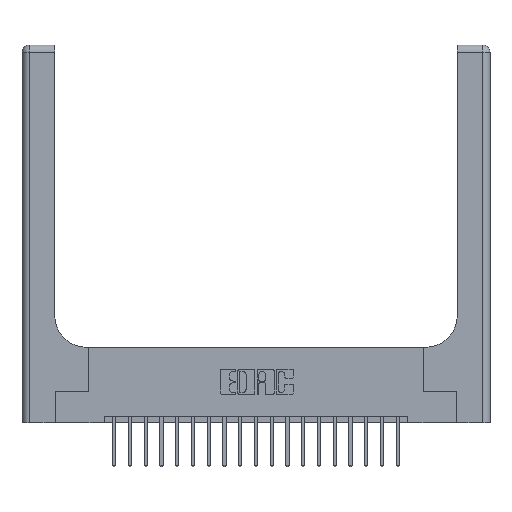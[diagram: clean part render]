
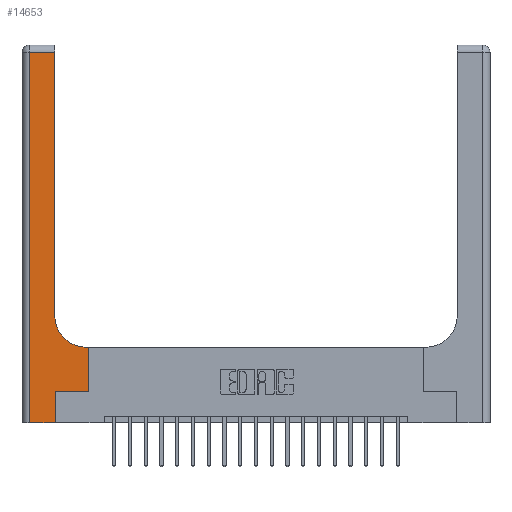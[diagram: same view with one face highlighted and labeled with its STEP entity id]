
A CAD part, top view. The second image highlights one B-rep face of the part: STEP entity #14653.
In plain terms, the highlighted planar face has unit normal (0, 0, 1).
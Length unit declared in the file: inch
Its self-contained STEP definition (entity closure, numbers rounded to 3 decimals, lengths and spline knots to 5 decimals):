
#74 = ORIENTED_EDGE ( 'NONE', *, *, #16744, .T. ) ;
#78 = AXIS2_PLACEMENT_3D ( 'NONE', #3815, #18214, #10391 ) ;
#103 = ORIENTED_EDGE ( 'NONE', *, *, #17492, .T. ) ;
#240 = VERTEX_POINT ( 'NONE', #12959 ) ;
#319 = CARTESIAN_POINT ( 'NONE',  ( 0., 3., 0.37 ) ) ;
#432 = LINE ( 'NONE', #9106, #1951 ) ;
#448 = ORIENTED_EDGE ( 'NONE', *, *, #4448, .T. ) ;
#1082 = ORIENTED_EDGE ( 'NONE', *, *, #11368, .T. ) ;
#1351 = CARTESIAN_POINT ( 'NONE',  ( 0.528, 0.25, 0.37 ) ) ;
#1389 = CARTESIAN_POINT ( 'NONE',  ( 0.06, 3., 0.37 ) ) ;
#1571 = CARTESIAN_POINT ( 'NONE',  ( 0.51, 0.6, 0.37 ) ) ;
#1824 = EDGE_CURVE ( 'NONE', #19904, #15926, #9438, .T. ) ;
#1832 = ORIENTED_EDGE ( 'NONE', *, *, #1824, .T. ) ;
#1951 = VECTOR ( 'NONE', #10669, 39.37008 ) ;
#2538 = CARTESIAN_POINT ( 'NONE',  ( 0.26, 2.94, 0.37 ) ) ;
#3023 = VERTEX_POINT ( 'NONE', #7259 ) ;
#3669 = EDGE_CURVE ( 'NONE', #5647, #3811, #8363, .T. ) ;
#3811 = VERTEX_POINT ( 'NONE', #5288 ) ;
#3815 = CARTESIAN_POINT ( 'NONE',  ( 0.51, 0.85, 0.37 ) ) ;
#4448 = EDGE_CURVE ( 'NONE', #3023, #19904, #19360, .T. ) ;
#4745 = VERTEX_POINT ( 'NONE', #18680 ) ;
#4746 = DIRECTION ( 'NONE',  ( -1., 0., 0. ) ) ;
#4914 = DIRECTION ( 'NONE',  ( 0., 0., -1. ) ) ;
#5176 = CARTESIAN_POINT ( 'NONE',  ( 0.265, 0.25, 0.37 ) ) ;
#5288 = CARTESIAN_POINT ( 'NONE',  ( 0.06, 2.94, 0.37 ) ) ;
#5647 = VERTEX_POINT ( 'NONE', #2538 ) ;
#5693 = ORIENTED_EDGE ( 'NONE', *, *, #3669, .T. ) ;
#6535 = DIRECTION ( 'NONE',  ( -1., 0., 0. ) ) ;
#6679 = CARTESIAN_POINT ( 'NONE',  ( 0.528, 0.25, 0.37 ) ) ;
#6680 = LINE ( 'NONE', #14009, #18183 ) ;
#7118 = VECTOR ( 'NONE', #4746, 39.37008 ) ;
#7122 = VECTOR ( 'NONE', #7865, 39.37008 ) ;
#7259 = CARTESIAN_POINT ( 'NONE',  ( 0.265, 0.25, 0.37 ) ) ;
#7482 = VERTEX_POINT ( 'NONE', #10153 ) ;
#7650 = EDGE_CURVE ( 'NONE', #11487, #240, #10318, .T. ) ;
#7865 = DIRECTION ( 'NONE',  ( 0., -1., 0. ) ) ;
#8240 = FACE_OUTER_BOUND ( 'NONE', #15623, .T. ) ;
#8363 = LINE ( 'NONE', #9780, #7118 ) ;
#8425 = VECTOR ( 'NONE', #17927, 39.37008 ) ;
#9106 = CARTESIAN_POINT ( 'NONE',  ( 0.265, 0., 0.37 ) ) ;
#9153 = CARTESIAN_POINT ( 'NONE',  ( 0.26, 3., 0.37 ) ) ;
#9438 = LINE ( 'NONE', #6679, #12708 ) ;
#9780 = CARTESIAN_POINT ( 'NONE',  ( 0., 2.94, 0.37 ) ) ;
#10153 = CARTESIAN_POINT ( 'NONE',  ( 0.06, 0., 0.37 ) ) ;
#10318 = CIRCLE ( 'NONE', #78, 0.25 ) ;
#10391 = DIRECTION ( 'NONE',  ( 1., 0., 0. ) ) ;
#10669 = DIRECTION ( 'NONE',  ( 0., 1., 0. ) ) ;
#10756 = EDGE_CURVE ( 'NONE', #240, #5647, #19450, .T. ) ;
#11368 = EDGE_CURVE ( 'NONE', #4745, #3023, #432, .T. ) ;
#11487 = VERTEX_POINT ( 'NONE', #1571 ) ;
#11767 = CARTESIAN_POINT ( 'NONE',  ( 0.26, 0.6, 0.37 ) ) ;
#12708 = VECTOR ( 'NONE', #17800, 39.37008 ) ;
#12905 = AXIS2_PLACEMENT_3D ( 'NONE', #319, #4914, #6535 ) ;
#12959 = CARTESIAN_POINT ( 'NONE',  ( 0.26, 0.85, 0.37 ) ) ;
#14009 = CARTESIAN_POINT ( 'NONE',  ( 0., 0., 0.37 ) ) ;
#14226 = LINE ( 'NONE', #11767, #8425 ) ;
#14653 = ADVANCED_FACE ( 'NONE', ( #8240 ), #17858, .F. ) ;
#14669 = CARTESIAN_POINT ( 'NONE',  ( 0.528, 0.6, 0.37 ) ) ;
#15095 = VECTOR ( 'NONE', #19467, 39.37008 ) ;
#15248 = ORIENTED_EDGE ( 'NONE', *, *, #7650, .T. ) ;
#15623 = EDGE_LOOP ( 'NONE', ( #17321, #5693, #16428, #103, #1082, #448, #1832, #74, #15248 ) ) ;
#15887 = LINE ( 'NONE', #1389, #7122 ) ;
#15926 = VERTEX_POINT ( 'NONE', #14669 ) ;
#16428 = ORIENTED_EDGE ( 'NONE', *, *, #18263, .T. ) ;
#16744 = EDGE_CURVE ( 'NONE', #15926, #11487, #14226, .T. ) ;
#17071 = DIRECTION ( 'NONE',  ( 1., 0., 0. ) ) ;
#17321 = ORIENTED_EDGE ( 'NONE', *, *, #10756, .T. ) ;
#17492 = EDGE_CURVE ( 'NONE', #7482, #4745, #6680, .T. ) ;
#17800 = DIRECTION ( 'NONE',  ( 0., 1., 0. ) ) ;
#17858 = PLANE ( 'NONE',  #12905 ) ;
#17927 = DIRECTION ( 'NONE',  ( -1., 0., 0. ) ) ;
#18183 = VECTOR ( 'NONE', #17071, 39.37008 ) ;
#18214 = DIRECTION ( 'NONE',  ( 0., 0., -1. ) ) ;
#18263 = EDGE_CURVE ( 'NONE', #3811, #7482, #15887, .T. ) ;
#18680 = CARTESIAN_POINT ( 'NONE',  ( 0.265, 0., 0.37 ) ) ;
#18823 = DIRECTION ( 'NONE',  ( 0., 1., 0. ) ) ;
#19360 = LINE ( 'NONE', #5176, #15095 ) ;
#19450 = LINE ( 'NONE', #9153, #20686 ) ;
#19467 = DIRECTION ( 'NONE',  ( 1., 0., 0. ) ) ;
#19904 = VERTEX_POINT ( 'NONE', #1351 ) ;
#20686 = VECTOR ( 'NONE', #18823, 39.37008 ) ;
